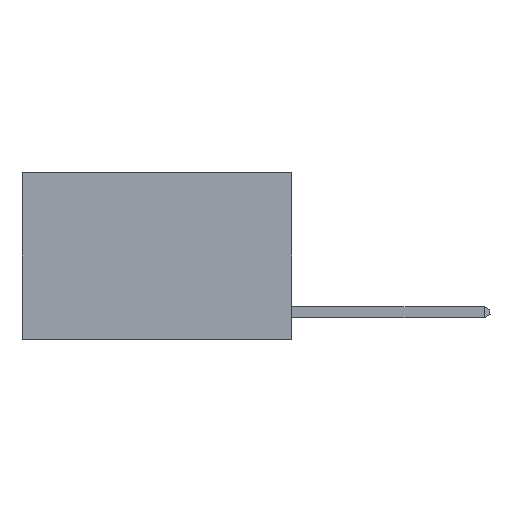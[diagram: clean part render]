
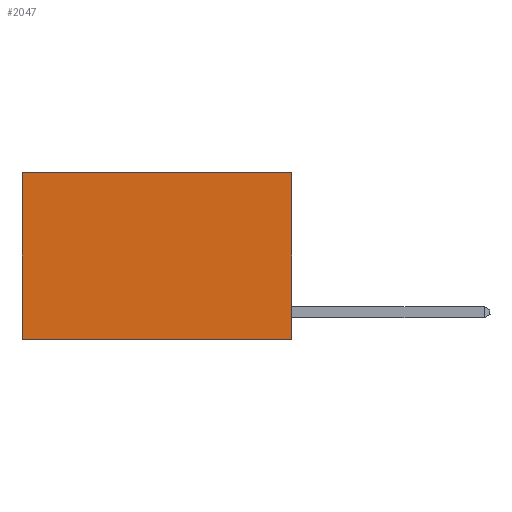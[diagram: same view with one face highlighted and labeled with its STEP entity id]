
A CAD part, left-side view. The second image highlights one B-rep face of the part: STEP entity #2047.
In plain terms, the highlighted planar face has unit normal (-1, 0, 0).
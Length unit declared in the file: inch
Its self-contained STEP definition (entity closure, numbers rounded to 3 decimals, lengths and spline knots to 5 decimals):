
#254 = CARTESIAN_POINT ( 'NONE',  ( 0.2625, 0., 0. ) ) ;
#2047 = ADVANCED_FACE ( 'NONE', ( #13371 ), #3871, .F. ) ;
#2373 = EDGE_CURVE ( 'NONE', #12473, #11538, #8806, .T. ) ;
#2518 = ORIENTED_EDGE ( 'NONE', *, *, #10167, .F. ) ;
#3752 = VECTOR ( 'NONE', #7571, 39.37008 ) ;
#3871 = PLANE ( 'NONE',  #12461 ) ;
#4170 = CARTESIAN_POINT ( 'NONE',  ( 0.2625, 0., -0.37 ) ) ;
#5347 = CARTESIAN_POINT ( 'NONE',  ( 0.2625, 0.6, -0.37 ) ) ;
#5750 = VECTOR ( 'NONE', #10604, 39.37008 ) ;
#6066 = DIRECTION ( 'NONE',  ( 0., 1., 0. ) ) ;
#6106 = VERTEX_POINT ( 'NONE', #9716 ) ;
#6213 = DIRECTION ( 'NONE',  ( 1., 0., 0. ) ) ;
#6394 = DIRECTION ( 'NONE',  ( 0., 1., 0. ) ) ;
#6921 = LINE ( 'NONE', #12754, #3752 ) ;
#7571 = DIRECTION ( 'NONE',  ( 0., 0., -1. ) ) ;
#7727 = VECTOR ( 'NONE', #6066, 39.37008 ) ;
#8151 = ORIENTED_EDGE ( 'NONE', *, *, #2373, .F. ) ;
#8286 = EDGE_CURVE ( 'NONE', #10579, #6106, #10812, .T. ) ;
#8524 = CARTESIAN_POINT ( 'NONE',  ( 0.2625, 0.6, 0. ) ) ;
#8806 = LINE ( 'NONE', #4170, #11237 ) ;
#9106 = CARTESIAN_POINT ( 'NONE',  ( 0.2625, 0., 0. ) ) ;
#9716 = CARTESIAN_POINT ( 'NONE',  ( 0.2625, 0.6, 0. ) ) ;
#10167 = EDGE_CURVE ( 'NONE', #10579, #12473, #6921, .T. ) ;
#10186 = EDGE_LOOP ( 'NONE', ( #10575, #8151, #2518, #14003 ) ) ;
#10575 = ORIENTED_EDGE ( 'NONE', *, *, #10785, .T. ) ;
#10579 = VERTEX_POINT ( 'NONE', #9106 ) ;
#10604 = DIRECTION ( 'NONE',  ( 0., 0., -1. ) ) ;
#10785 = EDGE_CURVE ( 'NONE', #6106, #11538, #14097, .T. ) ;
#10812 = LINE ( 'NONE', #254, #7727 ) ;
#11237 = VECTOR ( 'NONE', #6394, 39.37008 ) ;
#11426 = CARTESIAN_POINT ( 'NONE',  ( 0.2625, 0., 0. ) ) ;
#11538 = VERTEX_POINT ( 'NONE', #5347 ) ;
#12461 = AXIS2_PLACEMENT_3D ( 'NONE', #11426, #6213, #13575 ) ;
#12473 = VERTEX_POINT ( 'NONE', #12804 ) ;
#12754 = CARTESIAN_POINT ( 'NONE',  ( 0.2625, 0., 0. ) ) ;
#12804 = CARTESIAN_POINT ( 'NONE',  ( 0.2625, 0., -0.37 ) ) ;
#13371 = FACE_OUTER_BOUND ( 'NONE', #10186, .T. ) ;
#13575 = DIRECTION ( 'NONE',  ( 0., 0., -1. ) ) ;
#14003 = ORIENTED_EDGE ( 'NONE', *, *, #8286, .T. ) ;
#14097 = LINE ( 'NONE', #8524, #5750 ) ;
